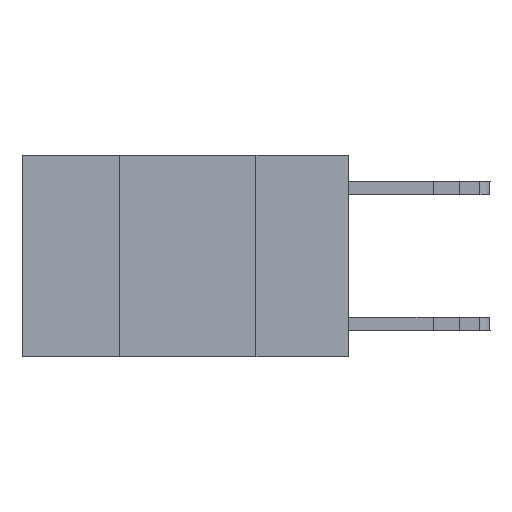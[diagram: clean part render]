
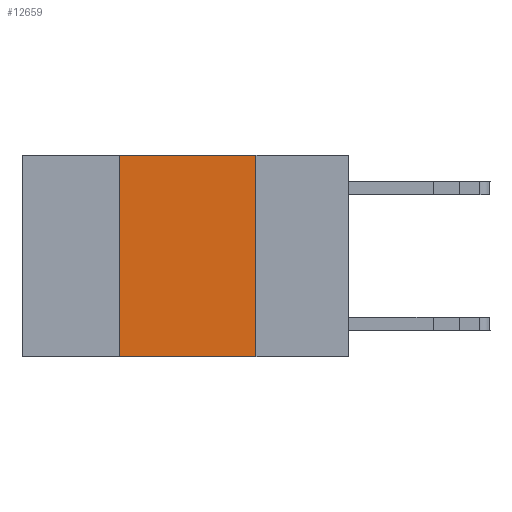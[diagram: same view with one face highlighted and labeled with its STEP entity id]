
A CAD part, left-side view. The second image highlights one B-rep face of the part: STEP entity #12659.
In plain terms, the highlighted planar face has unit normal (-1, 0, 0).
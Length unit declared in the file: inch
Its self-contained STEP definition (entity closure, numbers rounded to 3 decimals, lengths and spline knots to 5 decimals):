
#42 = CARTESIAN_POINT ( 'NONE',  ( 0., 0.6, -0.37 ) ) ;
#383 = CARTESIAN_POINT ( 'NONE',  ( 0., 0.6, 0. ) ) ;
#413 = LINE ( 'NONE', #42, #14247 ) ;
#533 = EDGE_CURVE ( 'NONE', #12594, #17808, #23502, .T. ) ;
#559 = EDGE_LOOP ( 'NONE', ( #2494, #3152, #12144, #21058 ) ) ;
#2494 = ORIENTED_EDGE ( 'NONE', *, *, #19307, .F. ) ;
#2959 = DIRECTION ( 'NONE',  ( 0., 0., 1. ) ) ;
#3152 = ORIENTED_EDGE ( 'NONE', *, *, #533, .F. ) ;
#4170 = CARTESIAN_POINT ( 'NONE',  ( 0., 0.17, 0. ) ) ;
#4352 = DIRECTION ( 'NONE',  ( 0., -1., 0. ) ) ;
#5501 = EDGE_CURVE ( 'NONE', #21431, #12594, #12457, .T. ) ;
#6172 = DIRECTION ( 'NONE',  ( 0., -1., 0. ) ) ;
#7517 = FACE_OUTER_BOUND ( 'NONE', #559, .T. ) ;
#7869 = VECTOR ( 'NONE', #23798, 39.37008 ) ;
#7882 = CARTESIAN_POINT ( 'NONE',  ( 0., 0.42, 0. ) ) ;
#9622 = DIRECTION ( 'NONE',  ( 0., 0., -1. ) ) ;
#10696 = CARTESIAN_POINT ( 'NONE',  ( 0., 0.42, 0. ) ) ;
#11865 = VERTEX_POINT ( 'NONE', #12020 ) ;
#12020 = CARTESIAN_POINT ( 'NONE',  ( 0., 0.17, -0.37 ) ) ;
#12086 = AXIS2_PLACEMENT_3D ( 'NONE', #19180, #13484, #9622 ) ;
#12144 = ORIENTED_EDGE ( 'NONE', *, *, #5501, .F. ) ;
#12457 = LINE ( 'NONE', #10696, #16663 ) ;
#12594 = VERTEX_POINT ( 'NONE', #7882 ) ;
#12626 = LINE ( 'NONE', #4170, #7869 ) ;
#12659 = ADVANCED_FACE ( 'NONE', ( #7517 ), #19051, .F. ) ;
#13135 = CARTESIAN_POINT ( 'NONE',  ( 0., 0.17, 0. ) ) ;
#13484 = DIRECTION ( 'NONE',  ( 1., 0., 0. ) ) ;
#14247 = VECTOR ( 'NONE', #6172, 39.37008 ) ;
#16663 = VECTOR ( 'NONE', #2959, 39.37008 ) ;
#17808 = VERTEX_POINT ( 'NONE', #13135 ) ;
#19051 = PLANE ( 'NONE',  #12086 ) ;
#19180 = CARTESIAN_POINT ( 'NONE',  ( 0., 0.6, 0. ) ) ;
#19307 = EDGE_CURVE ( 'NONE', #17808, #11865, #12626, .T. ) ;
#20053 = EDGE_CURVE ( 'NONE', #21431, #11865, #413, .T. ) ;
#20632 = VECTOR ( 'NONE', #4352, 39.37008 ) ;
#20923 = CARTESIAN_POINT ( 'NONE',  ( 0., 0.42, -0.37 ) ) ;
#21058 = ORIENTED_EDGE ( 'NONE', *, *, #20053, .T. ) ;
#21431 = VERTEX_POINT ( 'NONE', #20923 ) ;
#23502 = LINE ( 'NONE', #383, #20632 ) ;
#23798 = DIRECTION ( 'NONE',  ( 0., 0., -1. ) ) ;
